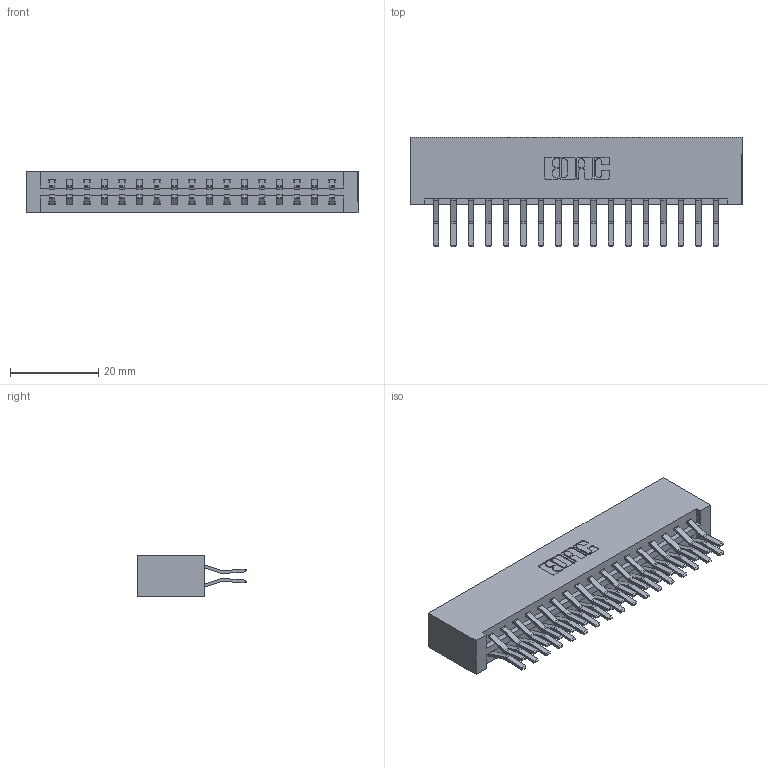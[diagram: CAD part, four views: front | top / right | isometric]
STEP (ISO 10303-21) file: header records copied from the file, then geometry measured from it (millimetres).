
FILE_DESCRIPTION (( 'STEP AP203' ), '1' );
FILE_NAME ('387-034-560-201.STEP', '2019-10-17T18:27:27', ( '' ), ( '' ), 'SwSTEP 2.0', 'SolidWorks 2016', '' );
FILE_SCHEMA (( 'CONFIG_CONTROL_DESIGN' ));
Length unit declared in the file: inch
Products named in the file (3): 337 Part_No Mounting Lugs; 387-034-560-201; 345-292-001_560 Tail
Assembly tree (35 placements, depth 2):
  387-034-560-201
    337 Part_No Mounting Lugs
    345-292-001_560 Tail  x34
Bounding box: 75.23 x 24.78 x 9.4 mm (x, y, z)
Volume: 8579.7 mm3; surface area: 10157.6 mm2
Topology: 35 solids, 35 shells, 2010 faces, 5965 edges, 3930 vertices
Faces by surface type: plane 1358, cylinder 652
Entity records: 16225 total; most frequent: CARTESIAN_POINT 2754, ORIENTED_EDGE 2690, DIRECTION 2385, EDGE_CURVE 1345, LINE 1221, VECTOR 1221, VERTEX_POINT 894, AXIS2_PLACEMENT_3D 582
